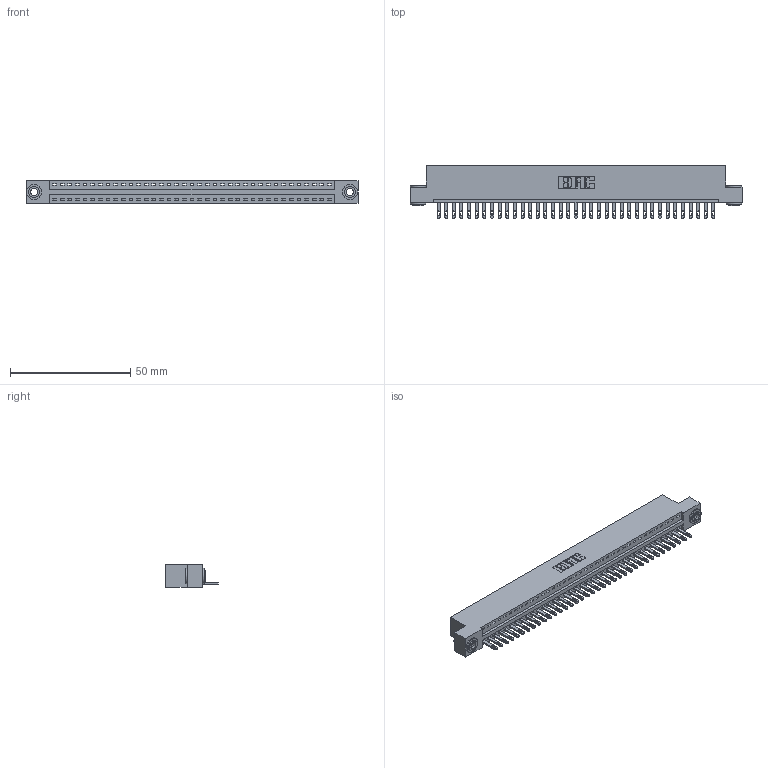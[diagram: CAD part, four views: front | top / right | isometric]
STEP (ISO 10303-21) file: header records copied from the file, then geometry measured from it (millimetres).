
FILE_DESCRIPTION (( 'STEP AP203' ), '1' );
FILE_NAME ('346-037-500-103.STEP', '2018-08-24T03:02:00', ( '' ), ( '' ), 'SwSTEP 2.0', 'SolidWorks 2016', '' );
FILE_SCHEMA (( 'CONFIG_CONTROL_DESIGN' ));
Length unit declared in the file: inch
Products named in the file (4): 346 Part_Flush Mounting Lugs - 0.156 Dia-TH; 345-292-001_345-293-100; 345-250-002_345-250-002-102; 346-037-500-103
Assembly tree (40 placements, depth 2):
  346-037-500-103
    346 Part_Flush Mounting Lugs - 0.156 Dia-TH
    345-292-001_345-293-100  x37
    345-250-002_345-250-002-102  x2
Bounding box: 138.05 x 21.84 x 9.4 mm (x, y, z)
Volume: 13222.2 mm3; surface area: 16777.5 mm2
Topology: 40 solids, 40 shells, 2158 faces, 6621 edges, 4410 vertices
Faces by surface type: plane 1344, cylinder 806, cone 8
Entity records: 24216 total; most frequent: CARTESIAN_POINT 4130, ORIENTED_EDGE 4094, DIRECTION 3683, EDGE_CURVE 2047, VECTOR 1739, LINE 1739, VERTEX_POINT 1362, AXIS2_PLACEMENT_3D 972
